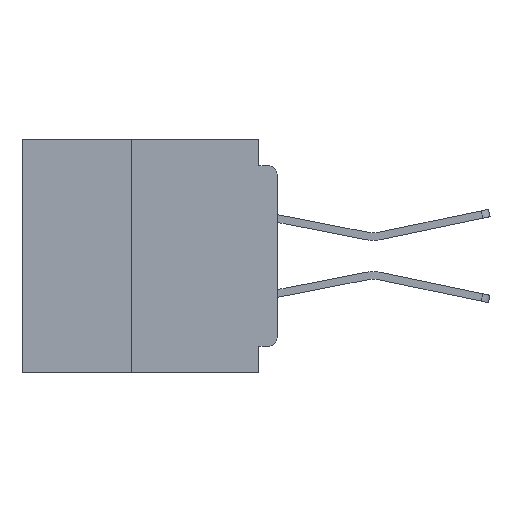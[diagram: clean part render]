
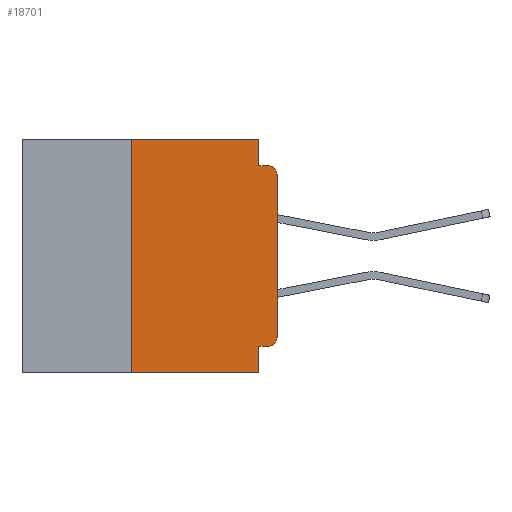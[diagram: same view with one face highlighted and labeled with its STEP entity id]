
A CAD part, left-side view. The second image highlights one B-rep face of the part: STEP entity #18701.
In plain terms, the highlighted planar face has unit normal (-1, 0, 0).
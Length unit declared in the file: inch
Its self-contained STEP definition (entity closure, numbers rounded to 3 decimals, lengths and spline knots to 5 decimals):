
#115 = CARTESIAN_POINT ( 'NONE',  ( 0., 0.015, -0.355 ) ) ;
#4167 = VECTOR ( 'NONE', #36439, 39.37008 ) ;
#4280 = CARTESIAN_POINT ( 'NONE',  ( 0., 0.25, -0.4 ) ) ;
#4543 = VERTEX_POINT ( 'NONE', #29319 ) ;
#5485 = VERTEX_POINT ( 'NONE', #8881 ) ;
#5546 = VECTOR ( 'NONE', #40608, 39.37008 ) ;
#8881 = CARTESIAN_POINT ( 'NONE',  ( 0., 0.25, 0. ) ) ;
#10473 = CARTESIAN_POINT ( 'NONE',  ( 0., 0.015, -0.34 ) ) ;
#10505 = CIRCLE ( 'NONE', #13705, 0.015 ) ;
#10952 = ORIENTED_EDGE ( 'NONE', *, *, #22772, .T. ) ;
#10972 = LINE ( 'NONE', #28274, #29128 ) ;
#10990 = CARTESIAN_POINT ( 'NONE',  ( 0., 0.031, -0.4 ) ) ;
#11149 = DIRECTION ( 'NONE',  ( 0., 0., -1. ) ) ;
#12912 = LINE ( 'NONE', #13725, #20339 ) ;
#13705 = AXIS2_PLACEMENT_3D ( 'NONE', #10473, #35832, #14159 ) ;
#13725 = CARTESIAN_POINT ( 'NONE',  ( 0., 0., 0. ) ) ;
#13915 = AXIS2_PLACEMENT_3D ( 'NONE', #42849, #21255, #46446 ) ;
#14159 = DIRECTION ( 'NONE',  ( 0., 0., -1. ) ) ;
#14406 = ORIENTED_EDGE ( 'NONE', *, *, #32536, .F. ) ;
#14781 = CARTESIAN_POINT ( 'NONE',  ( 0., 0.437, -0.4 ) ) ;
#14846 = CARTESIAN_POINT ( 'NONE',  ( 0., 0.031, -0.4 ) ) ;
#15126 = VERTEX_POINT ( 'NONE', #10990 ) ;
#15758 = EDGE_CURVE ( 'NONE', #22196, #15126, #34306, .T. ) ;
#16189 = CARTESIAN_POINT ( 'NONE',  ( 0., 0.031, 0. ) ) ;
#17784 = VECTOR ( 'NONE', #31055, 39.37008 ) ;
#18649 = CARTESIAN_POINT ( 'NONE',  ( 0., 0., -0.34 ) ) ;
#18701 = ADVANCED_FACE ( 'NONE', ( #42798 ), #20514, .F. ) ;
#19265 = LINE ( 'NONE', #16189, #37363 ) ;
#19604 = ORIENTED_EDGE ( 'NONE', *, *, #20177, .F. ) ;
#19836 = DIRECTION ( 'NONE',  ( 0., 0., -1. ) ) ;
#20061 = LINE ( 'NONE', #27433, #17784 ) ;
#20177 = EDGE_CURVE ( 'NONE', #32366, #15126, #20593, .T. ) ;
#20339 = VECTOR ( 'NONE', #24680, 39.37008 ) ;
#20514 = PLANE ( 'NONE',  #43456 ) ;
#20593 = LINE ( 'NONE', #14846, #38664 ) ;
#21148 = CARTESIAN_POINT ( 'NONE',  ( 0., 0.25, -0.4 ) ) ;
#21255 = DIRECTION ( 'NONE',  ( -1., 0., 0. ) ) ;
#21380 = VERTEX_POINT ( 'NONE', #32468 ) ;
#22196 = VERTEX_POINT ( 'NONE', #21148 ) ;
#22569 = EDGE_CURVE ( 'NONE', #21380, #4543, #19265, .T. ) ;
#22772 = EDGE_CURVE ( 'NONE', #41599, #26544, #37892, .T. ) ;
#23397 = EDGE_CURVE ( 'NONE', #28320, #41599, #12912, .T. ) ;
#24146 = DIRECTION ( 'NONE',  ( 0., 0., -1. ) ) ;
#24450 = EDGE_CURVE ( 'NONE', #28924, #32366, #20061, .T. ) ;
#24680 = DIRECTION ( 'NONE',  ( 0., 0., 1. ) ) ;
#25772 = ORIENTED_EDGE ( 'NONE', *, *, #22569, .F. ) ;
#26544 = VERTEX_POINT ( 'NONE', #33797 ) ;
#27433 = CARTESIAN_POINT ( 'NONE',  ( 0., 0., -0.355 ) ) ;
#28274 = CARTESIAN_POINT ( 'NONE',  ( 0., 0., -0.045 ) ) ;
#28320 = VERTEX_POINT ( 'NONE', #18649 ) ;
#28924 = VERTEX_POINT ( 'NONE', #115 ) ;
#29128 = VECTOR ( 'NONE', #46215, 39.37008 ) ;
#29319 = CARTESIAN_POINT ( 'NONE',  ( 0., 0.031, -0.045 ) ) ;
#29733 = ORIENTED_EDGE ( 'NONE', *, *, #15758, .T. ) ;
#30492 = CARTESIAN_POINT ( 'NONE',  ( 0., 0.437, 0. ) ) ;
#30790 = EDGE_CURVE ( 'NONE', #28924, #28320, #10505, .T. ) ;
#31055 = DIRECTION ( 'NONE',  ( 0., 1., 0. ) ) ;
#31232 = CARTESIAN_POINT ( 'NONE',  ( 0., 0.437, 0. ) ) ;
#31691 = VECTOR ( 'NONE', #33963, 39.37008 ) ;
#32366 = VERTEX_POINT ( 'NONE', #45272 ) ;
#32468 = CARTESIAN_POINT ( 'NONE',  ( 0., 0.031, 0. ) ) ;
#32536 = EDGE_CURVE ( 'NONE', #4543, #26544, #10972, .T. ) ;
#32614 = ORIENTED_EDGE ( 'NONE', *, *, #30790, .T. ) ;
#32827 = LINE ( 'NONE', #30492, #31691 ) ;
#33797 = CARTESIAN_POINT ( 'NONE',  ( 0., 0.015, -0.045 ) ) ;
#33963 = DIRECTION ( 'NONE',  ( 0., -1., 0. ) ) ;
#34180 = ORIENTED_EDGE ( 'NONE', *, *, #23397, .T. ) ;
#34306 = LINE ( 'NONE', #14781, #4167 ) ;
#34777 = CARTESIAN_POINT ( 'NONE',  ( 0., 0., -0.06 ) ) ;
#35112 = EDGE_LOOP ( 'NONE', ( #34180, #10952, #14406, #25772, #37653, #45510, #29733, #19604, #38826, #32614 ) ) ;
#35832 = DIRECTION ( 'NONE',  ( -1., 0., 0. ) ) ;
#36439 = DIRECTION ( 'NONE',  ( 0., -1., 0. ) ) ;
#37363 = VECTOR ( 'NONE', #19836, 39.37008 ) ;
#37653 = ORIENTED_EDGE ( 'NONE', *, *, #42154, .F. ) ;
#37892 = CIRCLE ( 'NONE', #13915, 0.015 ) ;
#38664 = VECTOR ( 'NONE', #11149, 39.37008 ) ;
#38826 = ORIENTED_EDGE ( 'NONE', *, *, #24450, .F. ) ;
#40608 = DIRECTION ( 'NONE',  ( 0., 0., 1. ) ) ;
#40690 = LINE ( 'NONE', #4280, #5546 ) ;
#41599 = VERTEX_POINT ( 'NONE', #34777 ) ;
#42154 = EDGE_CURVE ( 'NONE', #5485, #21380, #32827, .T. ) ;
#42798 = FACE_OUTER_BOUND ( 'NONE', #35112, .T. ) ;
#42849 = CARTESIAN_POINT ( 'NONE',  ( 0., 0.015, -0.06 ) ) ;
#43456 = AXIS2_PLACEMENT_3D ( 'NONE', #31232, #45701, #24146 ) ;
#45272 = CARTESIAN_POINT ( 'NONE',  ( 0., 0.031, -0.355 ) ) ;
#45510 = ORIENTED_EDGE ( 'NONE', *, *, #45895, .F. ) ;
#45701 = DIRECTION ( 'NONE',  ( 1., 0., 0. ) ) ;
#45895 = EDGE_CURVE ( 'NONE', #22196, #5485, #40690, .T. ) ;
#46215 = DIRECTION ( 'NONE',  ( 0., -1., 0. ) ) ;
#46446 = DIRECTION ( 'NONE',  ( 0., 0., -1. ) ) ;
